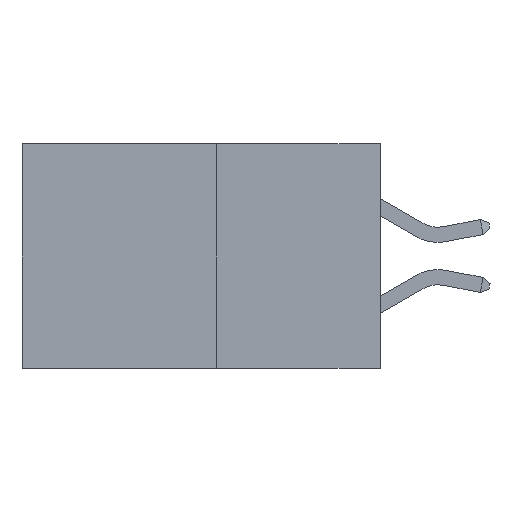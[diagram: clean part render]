
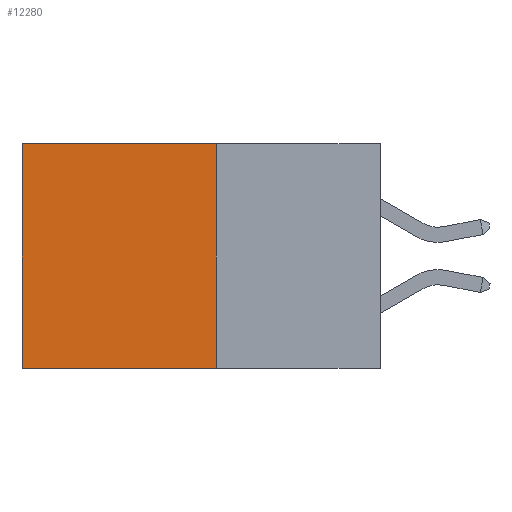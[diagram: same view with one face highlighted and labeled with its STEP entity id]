
A CAD part, left-side view. The second image highlights one B-rep face of the part: STEP entity #12280.
In plain terms, the highlighted planar face has unit normal (-1, 0, 0).
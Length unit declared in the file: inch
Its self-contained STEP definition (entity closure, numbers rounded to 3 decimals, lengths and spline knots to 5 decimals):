
#2552 = DIRECTION ( 'NONE',  ( 0., 0., -1. ) ) ;
#2714 = CARTESIAN_POINT ( 'NONE',  ( 0.277, 0.27, 0. ) ) ;
#2894 = FACE_OUTER_BOUND ( 'NONE', #15513, .T. ) ;
#4420 = VECTOR ( 'NONE', #4506, 39.37008 ) ;
#4506 = DIRECTION ( 'NONE',  ( 0., 1., 0. ) ) ;
#5023 = DIRECTION ( 'NONE',  ( 1., 0., 0. ) ) ;
#6533 = CARTESIAN_POINT ( 'NONE',  ( 0.277, 0.59, -0.37 ) ) ;
#8079 = EDGE_CURVE ( 'NONE', #10142, #12286, #17238, .T. ) ;
#8415 = CARTESIAN_POINT ( 'NONE',  ( 0.277, 0.59, 0. ) ) ;
#9257 = EDGE_CURVE ( 'NONE', #12286, #12999, #17449, .T. ) ;
#9572 = CARTESIAN_POINT ( 'NONE',  ( 0.277, 0.27, 0. ) ) ;
#9598 = DIRECTION ( 'NONE',  ( 0., 1., 0. ) ) ;
#10142 = VERTEX_POINT ( 'NONE', #9572 ) ;
#10327 = EDGE_CURVE ( 'NONE', #10142, #17993, #14338, .T. ) ;
#11516 = EDGE_CURVE ( 'NONE', #17993, #12999, #19976, .T. ) ;
#11665 = DIRECTION ( 'NONE',  ( 0., 0., -1. ) ) ;
#12206 = ORIENTED_EDGE ( 'NONE', *, *, #10327, .F. ) ;
#12280 = ADVANCED_FACE ( 'NONE', ( #2894 ), #18309, .F. ) ;
#12286 = VERTEX_POINT ( 'NONE', #8415 ) ;
#12858 = AXIS2_PLACEMENT_3D ( 'NONE', #15057, #5023, #16707 ) ;
#12944 = ORIENTED_EDGE ( 'NONE', *, *, #8079, .T. ) ;
#12999 = VERTEX_POINT ( 'NONE', #6533 ) ;
#13032 = VECTOR ( 'NONE', #2552, 39.37008 ) ;
#14338 = LINE ( 'NONE', #19920, #18209 ) ;
#14395 = CARTESIAN_POINT ( 'NONE',  ( 0.277, 0.59, -0.37 ) ) ;
#15057 = CARTESIAN_POINT ( 'NONE',  ( 0.277, 0.27, -0.37 ) ) ;
#15513 = EDGE_LOOP ( 'NONE', ( #21113, #19983, #12206, #12944 ) ) ;
#15936 = CARTESIAN_POINT ( 'NONE',  ( 0.277, 0.27, -0.37 ) ) ;
#16707 = DIRECTION ( 'NONE',  ( 0., 0., -1. ) ) ;
#17238 = LINE ( 'NONE', #2714, #4420 ) ;
#17449 = LINE ( 'NONE', #14395, #13032 ) ;
#17993 = VERTEX_POINT ( 'NONE', #15936 ) ;
#18209 = VECTOR ( 'NONE', #11665, 39.37008 ) ;
#18309 = PLANE ( 'NONE',  #12858 ) ;
#19920 = CARTESIAN_POINT ( 'NONE',  ( 0.277, 0.27, -0.37 ) ) ;
#19976 = LINE ( 'NONE', #21181, #21007 ) ;
#19983 = ORIENTED_EDGE ( 'NONE', *, *, #11516, .F. ) ;
#21007 = VECTOR ( 'NONE', #9598, 39.37008 ) ;
#21113 = ORIENTED_EDGE ( 'NONE', *, *, #9257, .T. ) ;
#21181 = CARTESIAN_POINT ( 'NONE',  ( 0.277, 0.27, -0.37 ) ) ;
